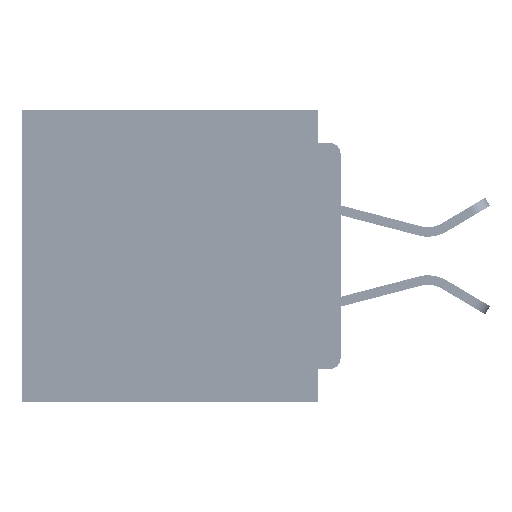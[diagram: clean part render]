
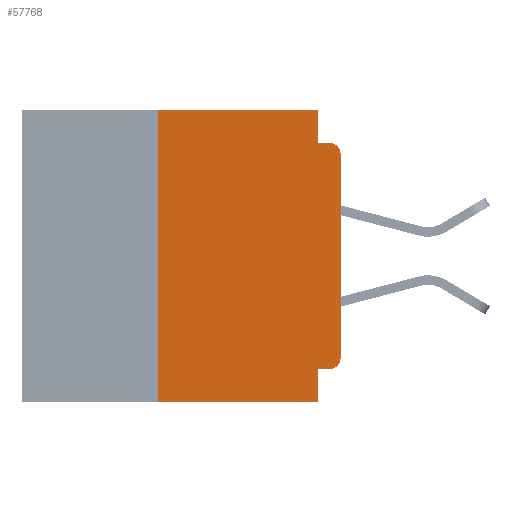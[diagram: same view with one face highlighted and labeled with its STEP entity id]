
A CAD part, left-side view. The second image highlights one B-rep face of the part: STEP entity #57768.
In plain terms, the highlighted planar face has unit normal (-1, 0, 0).
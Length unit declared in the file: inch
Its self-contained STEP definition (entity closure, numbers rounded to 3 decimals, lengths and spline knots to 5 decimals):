
#639 = EDGE_CURVE ( 'NONE', #66251, #21998, #40991, .T. ) ;
#1731 = VECTOR ( 'NONE', #30026, 39.37008 ) ;
#1888 = AXIS2_PLACEMENT_3D ( 'NONE', #9639, #46725, #14986 ) ;
#3571 = CARTESIAN_POINT ( 'NONE',  ( 0., 0.015, -0.355 ) ) ;
#4270 = CARTESIAN_POINT ( 'NONE',  ( 0., 0., -0.045 ) ) ;
#4842 = ORIENTED_EDGE ( 'NONE', *, *, #59230, .F. ) ;
#5230 = CARTESIAN_POINT ( 'NONE',  ( 0., 0.25, 0. ) ) ;
#9377 = LINE ( 'NONE', #60669, #22778 ) ;
#9379 = CARTESIAN_POINT ( 'NONE',  ( 0., 0.031, -0.4 ) ) ;
#9502 = VECTOR ( 'NONE', #60384, 39.37008 ) ;
#9639 = CARTESIAN_POINT ( 'NONE',  ( 0., 0.015, -0.06 ) ) ;
#11628 = CARTESIAN_POINT ( 'NONE',  ( 0., 0., -0.06 ) ) ;
#12227 = DIRECTION ( 'NONE',  ( 0., 0., -1. ) ) ;
#12535 = CIRCLE ( 'NONE', #1888, 0.015 ) ;
#12839 = LINE ( 'NONE', #34137, #9502 ) ;
#13844 = EDGE_CURVE ( 'NONE', #56759, #26900, #15860, .T. ) ;
#13929 = EDGE_CURVE ( 'NONE', #26900, #43918, #12535, .T. ) ;
#13959 = VERTEX_POINT ( 'NONE', #52447 ) ;
#14643 = VERTEX_POINT ( 'NONE', #42225 ) ;
#14968 = DIRECTION ( 'NONE',  ( 0., -1., 0. ) ) ;
#14986 = DIRECTION ( 'NONE',  ( 0., 0., -1. ) ) ;
#15860 = LINE ( 'NONE', #61347, #1731 ) ;
#17509 = EDGE_CURVE ( 'NONE', #25228, #14643, #12839, .T. ) ;
#18453 = DIRECTION ( 'NONE',  ( 0., 1., 0. ) ) ;
#19646 = EDGE_CURVE ( 'NONE', #61643, #21998, #32987, .T. ) ;
#20204 = ORIENTED_EDGE ( 'NONE', *, *, #57102, .T. ) ;
#21980 = ORIENTED_EDGE ( 'NONE', *, *, #26446, .F. ) ;
#21998 = VERTEX_POINT ( 'NONE', #9379 ) ;
#22133 = ORIENTED_EDGE ( 'NONE', *, *, #67778, .F. ) ;
#22778 = VECTOR ( 'NONE', #18453, 39.37008 ) ;
#23142 = DIRECTION ( 'NONE',  ( -1., 0., 0. ) ) ;
#24340 = DIRECTION ( 'NONE',  ( 0., 0., -1. ) ) ;
#24630 = CIRCLE ( 'NONE', #31543, 0.015 ) ;
#25228 = VERTEX_POINT ( 'NONE', #5230 ) ;
#26154 = ORIENTED_EDGE ( 'NONE', *, *, #13929, .T. ) ;
#26446 = EDGE_CURVE ( 'NONE', #37894, #61643, #9377, .T. ) ;
#26900 = VERTEX_POINT ( 'NONE', #11628 ) ;
#28843 = ORIENTED_EDGE ( 'NONE', *, *, #35777, .F. ) ;
#29416 = ORIENTED_EDGE ( 'NONE', *, *, #19646, .F. ) ;
#30026 = DIRECTION ( 'NONE',  ( 0., 0., 1. ) ) ;
#31543 = AXIS2_PLACEMENT_3D ( 'NONE', #54785, #23142, #60067 ) ;
#32987 = LINE ( 'NONE', #57778, #59351 ) ;
#33184 = ORIENTED_EDGE ( 'NONE', *, *, #13844, .T. ) ;
#33349 = PLANE ( 'NONE',  #53663 ) ;
#34137 = CARTESIAN_POINT ( 'NONE',  ( 0., 0.437, 0. ) ) ;
#35129 = ORIENTED_EDGE ( 'NONE', *, *, #639, .T. ) ;
#35245 = VECTOR ( 'NONE', #24340, 39.37008 ) ;
#35777 = EDGE_CURVE ( 'NONE', #13959, #43918, #54228, .T. ) ;
#36922 = DIRECTION ( 'NONE',  ( 0., 0., 1. ) ) ;
#37894 = VERTEX_POINT ( 'NONE', #3571 ) ;
#38532 = LINE ( 'NONE', #68444, #63188 ) ;
#38685 = CARTESIAN_POINT ( 'NONE',  ( 0., 0.437, 0. ) ) ;
#40243 = VECTOR ( 'NONE', #14968, 39.37008 ) ;
#40991 = LINE ( 'NONE', #62814, #53319 ) ;
#42162 = CARTESIAN_POINT ( 'NONE',  ( 0., 0.015, -0.045 ) ) ;
#42225 = CARTESIAN_POINT ( 'NONE',  ( 0., 0.031, 0. ) ) ;
#43918 = VERTEX_POINT ( 'NONE', #42162 ) ;
#44000 = DIRECTION ( 'NONE',  ( 1., 0., 0. ) ) ;
#44968 = ORIENTED_EDGE ( 'NONE', *, *, #17509, .F. ) ;
#46725 = DIRECTION ( 'NONE',  ( -1., 0., 0. ) ) ;
#50723 = CARTESIAN_POINT ( 'NONE',  ( 0., 0.25, -0.4 ) ) ;
#51842 = EDGE_LOOP ( 'NONE', ( #33184, #26154, #28843, #4842, #44968, #22133, #35129, #29416, #21980, #20204 ) ) ;
#52447 = CARTESIAN_POINT ( 'NONE',  ( 0., 0.031, -0.045 ) ) ;
#53319 = VECTOR ( 'NONE', #60634, 39.37008 ) ;
#53663 = AXIS2_PLACEMENT_3D ( 'NONE', #38685, #44000, #12227 ) ;
#54228 = LINE ( 'NONE', #4270, #40243 ) ;
#54785 = CARTESIAN_POINT ( 'NONE',  ( 0., 0.015, -0.34 ) ) ;
#55130 = FACE_OUTER_BOUND ( 'NONE', #51842, .T. ) ;
#56759 = VERTEX_POINT ( 'NONE', #62400 ) ;
#57102 = EDGE_CURVE ( 'NONE', #37894, #56759, #24630, .T. ) ;
#57768 = ADVANCED_FACE ( 'NONE', ( #55130 ), #33349, .F. ) ;
#57778 = CARTESIAN_POINT ( 'NONE',  ( 0., 0.031, -0.4 ) ) ;
#59230 = EDGE_CURVE ( 'NONE', #14643, #13959, #61590, .T. ) ;
#59351 = VECTOR ( 'NONE', #63034, 39.37008 ) ;
#59457 = CARTESIAN_POINT ( 'NONE',  ( 0., 0.031, -0.355 ) ) ;
#60067 = DIRECTION ( 'NONE',  ( 0., 0., -1. ) ) ;
#60384 = DIRECTION ( 'NONE',  ( 0., -1., 0. ) ) ;
#60634 = DIRECTION ( 'NONE',  ( 0., -1., 0. ) ) ;
#60669 = CARTESIAN_POINT ( 'NONE',  ( 0., 0., -0.355 ) ) ;
#61238 = CARTESIAN_POINT ( 'NONE',  ( 0., 0.031, 0. ) ) ;
#61347 = CARTESIAN_POINT ( 'NONE',  ( 0., 0., 0. ) ) ;
#61590 = LINE ( 'NONE', #61238, #35245 ) ;
#61643 = VERTEX_POINT ( 'NONE', #59457 ) ;
#62400 = CARTESIAN_POINT ( 'NONE',  ( 0., 0., -0.34 ) ) ;
#62814 = CARTESIAN_POINT ( 'NONE',  ( 0., 0.437, -0.4 ) ) ;
#63034 = DIRECTION ( 'NONE',  ( 0., 0., -1. ) ) ;
#63188 = VECTOR ( 'NONE', #36922, 39.37008 ) ;
#66251 = VERTEX_POINT ( 'NONE', #50723 ) ;
#67778 = EDGE_CURVE ( 'NONE', #66251, #25228, #38532, .T. ) ;
#68444 = CARTESIAN_POINT ( 'NONE',  ( 0., 0.25, -0.4 ) ) ;
